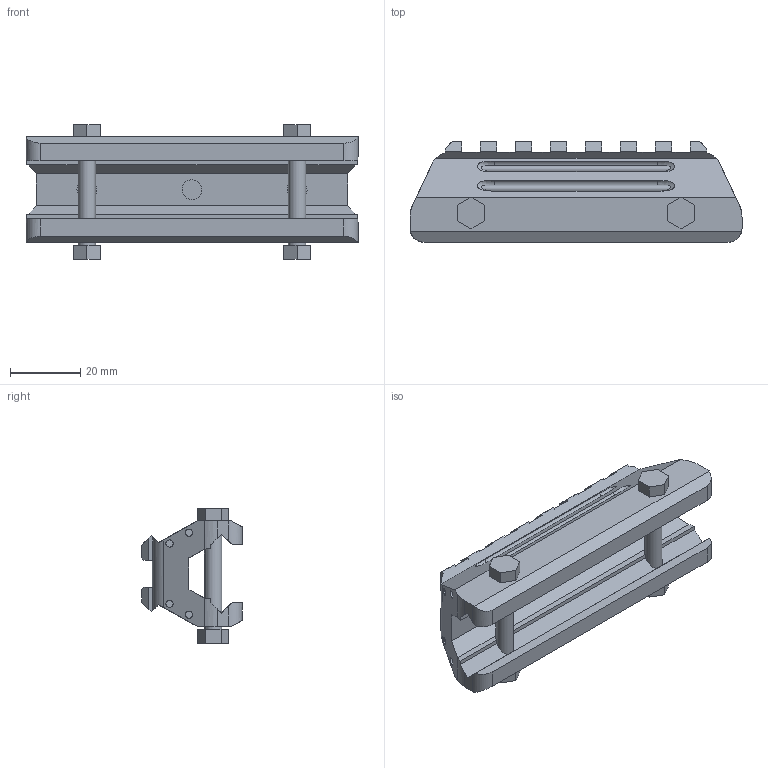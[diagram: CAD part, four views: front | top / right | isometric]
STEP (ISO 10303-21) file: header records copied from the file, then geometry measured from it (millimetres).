
FILE_DESCRIPTION(/* description */ (''),/* implementation_level */ '2;1');
FILE_NAME(/* name */ 'Sight Riser.step',/* time_stamp */ '2022-05-12T11:09:09-06:00',/* author */ (''),/* organization */ (''),/* preprocessor_version */ 'ST-DEVELOPER v18.1',/* originating_system */ 'Autodesk Translation Framework v10.10.0.1391',/* authorisation */ '');
FILE_SCHEMA (('AUTOMOTIVE_DESIGN { 1 0 10303 214 3 1 1 }'));
Length unit declared in the file: millimetre
Products named in the file (1): Sight riser
Bounding box: 94.75 x 28.68 x 38.5 mm (x, y, z)
Volume: 40460.9 mm3; surface area: 19557.1 mm2
Topology: 7 solids, 7 shells, 225 faces, 627 edges, 419 vertices
Faces by surface type: plane 185, cylinder 32, torus 8
Full cylindrical faces by diameter (mm): 2.05 x8, 4.97 x2, 5.2 x4
Entity records: 7596 total; most frequent: CARTESIAN_POINT 1624, ORIENTED_EDGE 1254, DIRECTION 1178, EDGE_CURVE 627, LINE 496, VECTOR 496, VERTEX_POINT 419, AXIS2_PLACEMENT_3D 341
